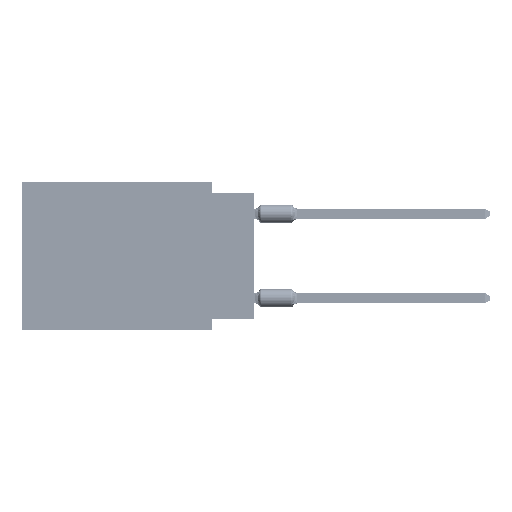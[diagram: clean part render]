
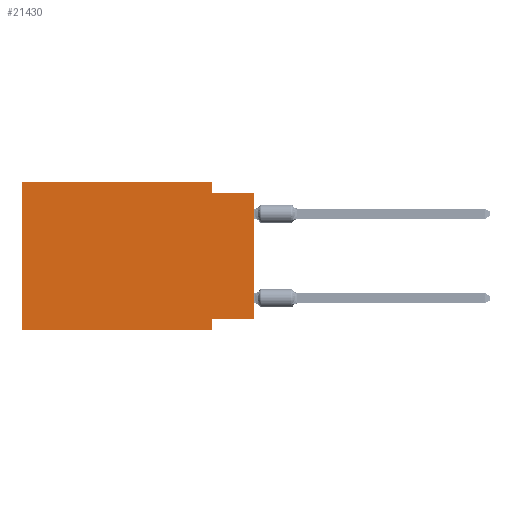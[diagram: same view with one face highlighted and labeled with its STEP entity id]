
A CAD part, left-side view. The second image highlights one B-rep face of the part: STEP entity #21430.
In plain terms, the highlighted planar face has unit normal (-1, 0, 0).
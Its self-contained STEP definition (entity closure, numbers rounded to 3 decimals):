
#116 = LINE ( 'NONE', #46635, #55300 ) ;
#147 = CARTESIAN_POINT ( 'NONE',  ( 0., 0., -0.635 ) ) ;
#3532 = DIRECTION ( 'NONE',  ( 0., 0., -1. ) ) ;
#3695 = CARTESIAN_POINT ( 'NONE',  ( 0., 13.97, -8.89 ) ) ;
#3847 = EDGE_LOOP ( 'NONE', ( #18691, #23562, #43094, #23371, #54149, #60457, #32463, #36430 ) ) ;
#3888 = CARTESIAN_POINT ( 'NONE',  ( 0., 2.54, -8.89 ) ) ;
#5285 = DIRECTION ( 'NONE',  ( 0., -1., 0. ) ) ;
#7390 = CARTESIAN_POINT ( 'NONE',  ( 0., 2.54, 0. ) ) ;
#8003 = VECTOR ( 'NONE', #36166, 1000. ) ;
#9333 = CARTESIAN_POINT ( 'NONE',  ( 0., 0., 0. ) ) ;
#12388 = VERTEX_POINT ( 'NONE', #21155 ) ;
#16123 = LINE ( 'NONE', #36971, #28919 ) ;
#18691 = ORIENTED_EDGE ( 'NONE', *, *, #51128, .T. ) ;
#18919 = LINE ( 'NONE', #9333, #43985 ) ;
#21155 = CARTESIAN_POINT ( 'NONE',  ( 0., 0., -8.255 ) ) ;
#21257 = DIRECTION ( 'NONE',  ( 0., 0., 1. ) ) ;
#21430 = ADVANCED_FACE ( 'NONE', ( #39235 ), #23528, .F. ) ;
#23371 = ORIENTED_EDGE ( 'NONE', *, *, #57424, .F. ) ;
#23528 = PLANE ( 'NONE',  #29774 ) ;
#23562 = ORIENTED_EDGE ( 'NONE', *, *, #42000, .F. ) ;
#23751 = EDGE_CURVE ( 'NONE', #25305, #37707, #16123, .T. ) ;
#24070 = VERTEX_POINT ( 'NONE', #30753 ) ;
#24726 = DIRECTION ( 'NONE',  ( 0., 0., 1. ) ) ;
#25305 = VERTEX_POINT ( 'NONE', #36722 ) ;
#25432 = DIRECTION ( 'NONE',  ( 0., 0., -1. ) ) ;
#26126 = VERTEX_POINT ( 'NONE', #7390 ) ;
#26772 = CARTESIAN_POINT ( 'NONE',  ( 0., 0., -8.255 ) ) ;
#28919 = VECTOR ( 'NONE', #21257, 1000. ) ;
#29774 = AXIS2_PLACEMENT_3D ( 'NONE', #61081, #49504, #66206 ) ;
#29893 = LINE ( 'NONE', #50745, #42167 ) ;
#30638 = VECTOR ( 'NONE', #3532, 1000. ) ;
#30753 = CARTESIAN_POINT ( 'NONE',  ( 0., 2.54, -8.89 ) ) ;
#32229 = VERTEX_POINT ( 'NONE', #52404 ) ;
#32381 = VERTEX_POINT ( 'NONE', #47942 ) ;
#32463 = ORIENTED_EDGE ( 'NONE', *, *, #45271, .F. ) ;
#34972 = EDGE_CURVE ( 'NONE', #26126, #32229, #29893, .T. ) ;
#36166 = DIRECTION ( 'NONE',  ( 0., -1., 0. ) ) ;
#36430 = ORIENTED_EDGE ( 'NONE', *, *, #61675, .F. ) ;
#36722 = CARTESIAN_POINT ( 'NONE',  ( 0., 13.97, -8.89 ) ) ;
#36971 = CARTESIAN_POINT ( 'NONE',  ( 0., 13.97, 0. ) ) ;
#37281 = CARTESIAN_POINT ( 'NONE',  ( 0., 2.54, -8.255 ) ) ;
#37707 = VERTEX_POINT ( 'NONE', #66088 ) ;
#39235 = FACE_OUTER_BOUND ( 'NONE', #3847, .T. ) ;
#39432 = VERTEX_POINT ( 'NONE', #37281 ) ;
#41352 = VECTOR ( 'NONE', #63333, 1000. ) ;
#42000 = EDGE_CURVE ( 'NONE', #32229, #32381, #57597, .T. ) ;
#42167 = VECTOR ( 'NONE', #25432, 1000. ) ;
#43094 = ORIENTED_EDGE ( 'NONE', *, *, #34972, .F. ) ;
#43985 = VECTOR ( 'NONE', #24726, 1000. ) ;
#45271 = EDGE_CURVE ( 'NONE', #39432, #24070, #50384, .T. ) ;
#46635 = CARTESIAN_POINT ( 'NONE',  ( 0., 13.97, 0. ) ) ;
#47942 = CARTESIAN_POINT ( 'NONE',  ( 0., 0., -0.635 ) ) ;
#49504 = DIRECTION ( 'NONE',  ( 1., 0., 0. ) ) ;
#49741 = VECTOR ( 'NONE', #5285, 1000. ) ;
#50384 = LINE ( 'NONE', #3888, #30638 ) ;
#50745 = CARTESIAN_POINT ( 'NONE',  ( 0., 2.54, 0. ) ) ;
#51128 = EDGE_CURVE ( 'NONE', #12388, #32381, #18919, .T. ) ;
#51957 = EDGE_CURVE ( 'NONE', #25305, #24070, #55681, .T. ) ;
#52079 = LINE ( 'NONE', #26772, #41352 ) ;
#52404 = CARTESIAN_POINT ( 'NONE',  ( 0., 2.54, -0.635 ) ) ;
#54149 = ORIENTED_EDGE ( 'NONE', *, *, #23751, .F. ) ;
#55300 = VECTOR ( 'NONE', #67473, 1000. ) ;
#55681 = LINE ( 'NONE', #3695, #8003 ) ;
#57424 = EDGE_CURVE ( 'NONE', #37707, #26126, #116, .T. ) ;
#57597 = LINE ( 'NONE', #147, #49741 ) ;
#60457 = ORIENTED_EDGE ( 'NONE', *, *, #51957, .T. ) ;
#61081 = CARTESIAN_POINT ( 'NONE',  ( 0., 13.97, 0. ) ) ;
#61675 = EDGE_CURVE ( 'NONE', #12388, #39432, #52079, .T. ) ;
#63333 = DIRECTION ( 'NONE',  ( 0., 1., 0. ) ) ;
#66088 = CARTESIAN_POINT ( 'NONE',  ( 0., 13.97, 0. ) ) ;
#66206 = DIRECTION ( 'NONE',  ( 0., 0., -1. ) ) ;
#67473 = DIRECTION ( 'NONE',  ( 0., -1., 0. ) ) ;
